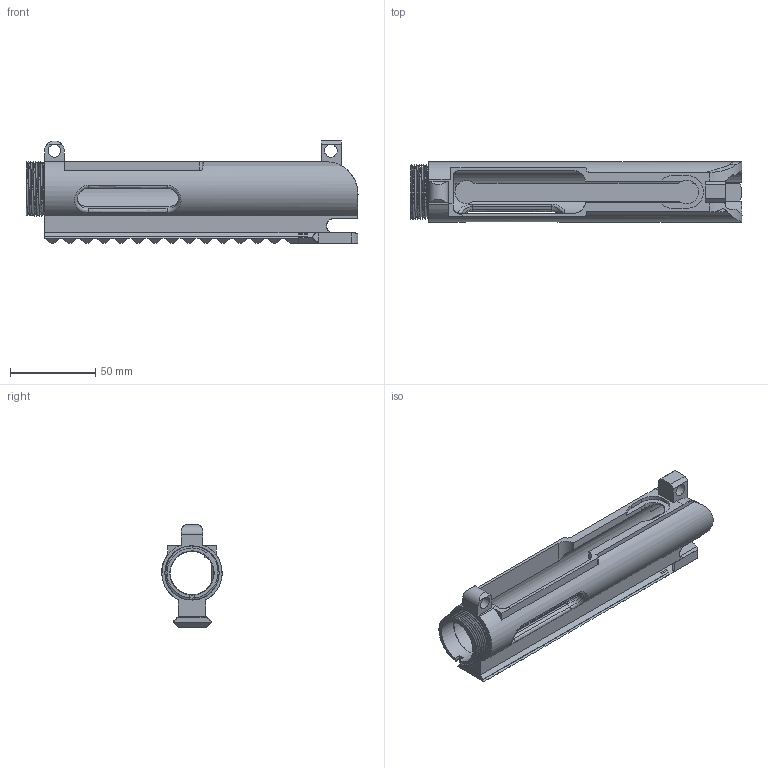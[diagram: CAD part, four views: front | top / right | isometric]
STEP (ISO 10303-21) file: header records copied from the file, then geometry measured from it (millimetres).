
FILE_DESCRIPTION(/* description */ (''),/* implementation_level */ '2;1');
FILE_NAME(/* name */ 'Tubee-22 UPPER FINAL.step',/* time_stamp */ '2021-07-12T16:01:41-04:00',/* author */ (''),/* organization */ (''),/* preprocessor_version */ 'ST-DEVELOPER v18.1',/* originating_system */ 'Autodesk Translation Framework v10.9.0.1377',/* authorisation */ '');
FILE_SCHEMA (('AUTOMOTIVE_DESIGN { 1 0 10303 214 3 1 1 }','AP242_MANAGED_MODEL_BASED_3D_ENGINEERING_MIM_LF { 1 0 10303 442 1 1 4 }'));
Length unit declared in the file: millimetre
Products named in the file (3): (Unsaved); AR22 v11.step; Upper, Core
Assembly tree (2 placements, depth 3):
  (Unsaved)
    AR22 v11.step
      Upper, Core
Bounding box: 194.4 x 35.24 x 59.97 mm (x, y, z)
Volume: 84420.8 mm3; surface area: 49238.8 mm2
Topology: 1 solids, 2 shells, 600 faces, 1663 edges, 1071 vertices
Faces by surface type: plane 296, bspline 172, cylinder 81, cone 48, torus 3
Full cylindrical faces by diameter (mm): 7.35 x1, 7.358 x1, 25.546 x1, 25.927 x1, 29.782 x1, 31.7 x4
Entity records: 23111 total; most frequent: CARTESIAN_POINT 9060, ORIENTED_EDGE 3324, DIRECTION 2235, EDGE_CURVE 1662, VERTEX_POINT 1071, LINE 971, VECTOR 971, AXIS2_PLACEMENT_3D 632
